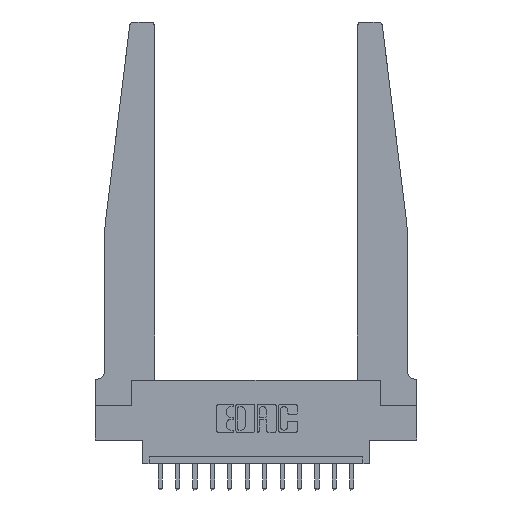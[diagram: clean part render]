
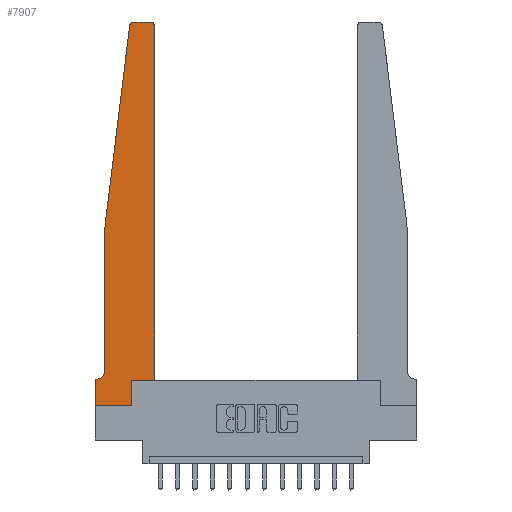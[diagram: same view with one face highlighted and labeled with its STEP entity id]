
A CAD part, top view. The second image highlights one B-rep face of the part: STEP entity #7907.
In plain terms, the highlighted planar face has unit normal (0, 0, 1).
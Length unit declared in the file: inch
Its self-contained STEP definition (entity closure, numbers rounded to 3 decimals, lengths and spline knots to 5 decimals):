
#14 = LINE ( 'NONE', #15943, #7656 ) ;
#22 = LINE ( 'NONE', #12650, #8802 ) ;
#95 = CARTESIAN_POINT ( 'NONE',  ( 0., 0., 0.37 ) ) ;
#322 = CARTESIAN_POINT ( 'NONE',  ( 0.425, 0.18, 0.37 ) ) ;
#733 = LINE ( 'NONE', #5511, #15070 ) ;
#826 = CARTESIAN_POINT ( 'NONE',  ( 0.065, 1.25, 0.37 ) ) ;
#1046 = CARTESIAN_POINT ( 'NONE',  ( 0.24675, 2.72367, 0.37 ) ) ;
#1048 = EDGE_CURVE ( 'NONE', #14366, #9022, #3662, .T. ) ;
#1479 = VERTEX_POINT ( 'NONE', #3772 ) ;
#1509 = DIRECTION ( 'NONE',  ( -1., 0., 0. ) ) ;
#1778 = EDGE_LOOP ( 'NONE', ( #4975, #8457, #5266, #12970, #8671, #13426, #9270, #5733, #15638, #8966, #12083, #4557 ) ) ;
#1987 = DIRECTION ( 'NONE',  ( 0., 1., 0. ) ) ;
#2173 = AXIS2_PLACEMENT_3D ( 'NONE', #3939, #3888, #14093 ) ;
#2222 = EDGE_CURVE ( 'NONE', #2347, #1479, #14, .T. ) ;
#2271 = DIRECTION ( 'NONE',  ( 1., 0., 0. ) ) ;
#2347 = VERTEX_POINT ( 'NONE', #9950 ) ;
#2595 = CARTESIAN_POINT ( 'NONE',  ( 0., 0.1875, 0.37 ) ) ;
#2630 = LINE ( 'NONE', #322, #7180 ) ;
#2685 = CARTESIAN_POINT ( 'NONE',  ( 0.015, 0.1875, 0.37 ) ) ;
#2946 = CARTESIAN_POINT ( 'NONE',  ( 0.065, 0.2375, 0.37 ) ) ;
#2978 = LINE ( 'NONE', #4053, #8709 ) ;
#3167 = CARTESIAN_POINT ( 'NONE',  ( 0., 0., 0.37 ) ) ;
#3662 = LINE ( 'NONE', #11615, #14589 ) ;
#3772 = CARTESIAN_POINT ( 'NONE',  ( 0.425, 2.72, 0.37 ) ) ;
#3888 = DIRECTION ( 'NONE',  ( 0., 0., 1. ) ) ;
#3939 = CARTESIAN_POINT ( 'NONE',  ( 0.395, 2.72, 0.37 ) ) ;
#4053 = CARTESIAN_POINT ( 'NONE',  ( 0.25, 2.75, 0.37 ) ) ;
#4067 = CARTESIAN_POINT ( 'NONE',  ( 0.065, 1.25, 0.37 ) ) ;
#4160 = EDGE_CURVE ( 'NONE', #5499, #15633, #8315, .T. ) ;
#4557 = ORIENTED_EDGE ( 'NONE', *, *, #11154, .T. ) ;
#4631 = CARTESIAN_POINT ( 'NONE',  ( 0.2605, 0.18, 0.37 ) ) ;
#4975 = ORIENTED_EDGE ( 'NONE', *, *, #13631, .T. ) ;
#5263 = DIRECTION ( 'NONE',  ( 0., 0., 1. ) ) ;
#5266 = ORIENTED_EDGE ( 'NONE', *, *, #11681, .T. ) ;
#5499 = VERTEX_POINT ( 'NONE', #6817 ) ;
#5511 = CARTESIAN_POINT ( 'NONE',  ( 0.065, 1.25, 0.37 ) ) ;
#5530 = DIRECTION ( 'NONE',  ( -1., 0., 0. ) ) ;
#5614 = CARTESIAN_POINT ( 'NONE',  ( 0.015, 0.2375, 0.37 ) ) ;
#5733 = ORIENTED_EDGE ( 'NONE', *, *, #12287, .T. ) ;
#5840 = AXIS2_PLACEMENT_3D ( 'NONE', #15250, #15376, #10343 ) ;
#6098 = EDGE_CURVE ( 'NONE', #10902, #14366, #11072, .T. ) ;
#6526 = EDGE_CURVE ( 'NONE', #15230, #14737, #22, .T. ) ;
#6807 = VERTEX_POINT ( 'NONE', #10140 ) ;
#6817 = CARTESIAN_POINT ( 'NONE',  ( 0.27653, 2.75, 0.37 ) ) ;
#7003 = LINE ( 'NONE', #826, #7614 ) ;
#7180 = VECTOR ( 'NONE', #15458, 39.37008 ) ;
#7576 = DIRECTION ( 'NONE',  ( 0., -1., 0. ) ) ;
#7614 = VECTOR ( 'NONE', #15016, 39.37008 ) ;
#7656 = VECTOR ( 'NONE', #1987, 39.37008 ) ;
#7665 = DIRECTION ( 'NONE',  ( 0., 1., 0. ) ) ;
#7907 = ADVANCED_FACE ( 'NONE', ( #14942 ), #12866, .T. ) ;
#7962 = DIRECTION ( 'NONE',  ( 0., 0., -1. ) ) ;
#8315 = CIRCLE ( 'NONE', #5840, 0.03 ) ;
#8457 = ORIENTED_EDGE ( 'NONE', *, *, #4160, .T. ) ;
#8671 = ORIENTED_EDGE ( 'NONE', *, *, #6098, .T. ) ;
#8709 = VECTOR ( 'NONE', #1509, 39.37008 ) ;
#8802 = VECTOR ( 'NONE', #7665, 39.37008 ) ;
#8966 = ORIENTED_EDGE ( 'NONE', *, *, #11876, .T. ) ;
#9022 = VERTEX_POINT ( 'NONE', #13597 ) ;
#9270 = ORIENTED_EDGE ( 'NONE', *, *, #13091, .T. ) ;
#9332 = VERTEX_POINT ( 'NONE', #4067 ) ;
#9837 = VERTEX_POINT ( 'NONE', #3167 ) ;
#9950 = CARTESIAN_POINT ( 'NONE',  ( 0.425, 0.18, 0.37 ) ) ;
#10132 = AXIS2_PLACEMENT_3D ( 'NONE', #5614, #7962, #15728 ) ;
#10140 = CARTESIAN_POINT ( 'NONE',  ( 0.395, 2.75, 0.37 ) ) ;
#10343 = DIRECTION ( 'NONE',  ( 1., 0., 0. ) ) ;
#10885 = DIRECTION ( 'NONE',  ( 0., -1., 0. ) ) ;
#10902 = VERTEX_POINT ( 'NONE', #2946 ) ;
#11072 = CIRCLE ( 'NONE', #10132, 0.05 ) ;
#11154 = EDGE_CURVE ( 'NONE', #1479, #6807, #11232, .T. ) ;
#11232 = CIRCLE ( 'NONE', #2173, 0.03 ) ;
#11494 = DIRECTION ( 'NONE',  ( 1., 0., 0. ) ) ;
#11615 = CARTESIAN_POINT ( 'NONE',  ( 0.065, 0.1875, 0.37 ) ) ;
#11681 = EDGE_CURVE ( 'NONE', #15633, #9332, #7003, .T. ) ;
#11876 = EDGE_CURVE ( 'NONE', #14737, #2347, #2630, .T. ) ;
#12083 = ORIENTED_EDGE ( 'NONE', *, *, #2222, .T. ) ;
#12287 = EDGE_CURVE ( 'NONE', #9837, #15230, #13938, .T. ) ;
#12650 = CARTESIAN_POINT ( 'NONE',  ( 0.2605, 0.18, 0.37 ) ) ;
#12800 = AXIS2_PLACEMENT_3D ( 'NONE', #2595, #5263, #11494 ) ;
#12866 = PLANE ( 'NONE',  #12800 ) ;
#12924 = VECTOR ( 'NONE', #7576, 39.37008 ) ;
#12970 = ORIENTED_EDGE ( 'NONE', *, *, #13880, .T. ) ;
#13091 = EDGE_CURVE ( 'NONE', #9022, #9837, #13524, .T. ) ;
#13426 = ORIENTED_EDGE ( 'NONE', *, *, #1048, .T. ) ;
#13524 = LINE ( 'NONE', #95, #12924 ) ;
#13597 = CARTESIAN_POINT ( 'NONE',  ( 0., 0.1875, 0.37 ) ) ;
#13631 = EDGE_CURVE ( 'NONE', #6807, #5499, #2978, .T. ) ;
#13880 = EDGE_CURVE ( 'NONE', #9332, #10902, #733, .T. ) ;
#13938 = LINE ( 'NONE', #14994, #14749 ) ;
#14093 = DIRECTION ( 'NONE',  ( 1., 0., 0. ) ) ;
#14366 = VERTEX_POINT ( 'NONE', #2685 ) ;
#14589 = VECTOR ( 'NONE', #5530, 39.37008 ) ;
#14737 = VERTEX_POINT ( 'NONE', #4631 ) ;
#14749 = VECTOR ( 'NONE', #2271, 39.37008 ) ;
#14942 = FACE_OUTER_BOUND ( 'NONE', #1778, .T. ) ;
#14994 = CARTESIAN_POINT ( 'NONE',  ( 0., 0., 0.37 ) ) ;
#15016 = DIRECTION ( 'NONE',  ( -0.122, -0.992, 0. ) ) ;
#15070 = VECTOR ( 'NONE', #10885, 39.37008 ) ;
#15230 = VERTEX_POINT ( 'NONE', #16256 ) ;
#15250 = CARTESIAN_POINT ( 'NONE',  ( 0.27653, 2.72, 0.37 ) ) ;
#15376 = DIRECTION ( 'NONE',  ( 0., 0., 1. ) ) ;
#15458 = DIRECTION ( 'NONE',  ( 1., 0., 0. ) ) ;
#15633 = VERTEX_POINT ( 'NONE', #1046 ) ;
#15638 = ORIENTED_EDGE ( 'NONE', *, *, #6526, .T. ) ;
#15728 = DIRECTION ( 'NONE',  ( -1., 0., 0. ) ) ;
#15943 = CARTESIAN_POINT ( 'NONE',  ( 0.425, 0.18, 0.37 ) ) ;
#16256 = CARTESIAN_POINT ( 'NONE',  ( 0.2605, 0., 0.37 ) ) ;
